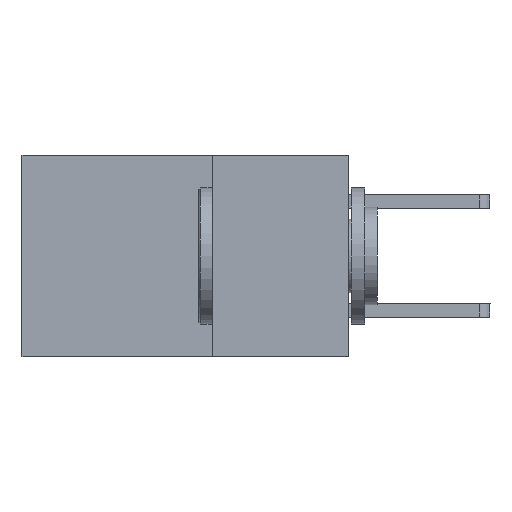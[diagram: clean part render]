
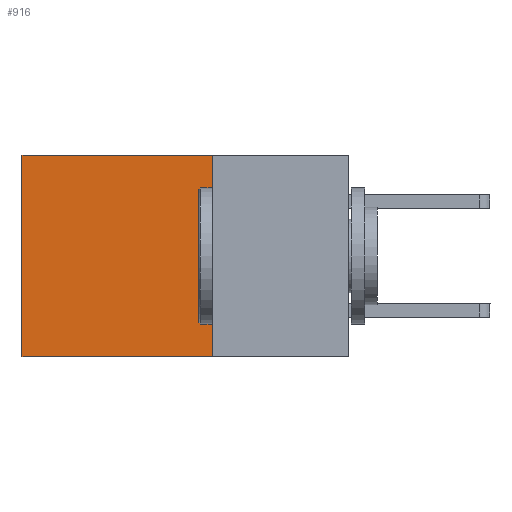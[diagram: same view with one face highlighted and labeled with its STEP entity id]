
A CAD part, left-side view. The second image highlights one B-rep face of the part: STEP entity #916.
In plain terms, the highlighted planar face has unit normal (-1, 0, 0).
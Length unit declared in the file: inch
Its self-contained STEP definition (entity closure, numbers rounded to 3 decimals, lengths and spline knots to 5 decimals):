
#93 = ORIENTED_EDGE ( 'NONE', *, *, #2616, .F. ) ;
#195 = CARTESIAN_POINT ( 'NONE',  ( 0.298, 0.25, 0. ) ) ;
#203 = LINE ( 'NONE', #5521, #3733 ) ;
#425 = VERTEX_POINT ( 'NONE', #1299 ) ;
#738 = DIRECTION ( 'NONE',  ( 0., 0., -1. ) ) ;
#740 = VERTEX_POINT ( 'NONE', #9768 ) ;
#897 = VECTOR ( 'NONE', #2485, 39.37008 ) ;
#916 = ADVANCED_FACE ( 'NONE', ( #6773 ), #8336, .F. ) ;
#918 = VECTOR ( 'NONE', #9414, 39.37008 ) ;
#1045 = DIRECTION ( 'NONE',  ( 0., 0., -1. ) ) ;
#1299 = CARTESIAN_POINT ( 'NONE',  ( 0.298, 0.25, -0.37 ) ) ;
#1540 = CARTESIAN_POINT ( 'NONE',  ( 0.298, 0.25, 0. ) ) ;
#1793 = VECTOR ( 'NONE', #9292, 39.37008 ) ;
#2485 = DIRECTION ( 'NONE',  ( 0., 0., -1. ) ) ;
#2616 = EDGE_CURVE ( 'NONE', #8647, #425, #4197, .T. ) ;
#3731 = CARTESIAN_POINT ( 'NONE',  ( 0.298, 0.25, 0. ) ) ;
#3733 = VECTOR ( 'NONE', #738, 39.37008 ) ;
#3848 = ORIENTED_EDGE ( 'NONE', *, *, #5344, .F. ) ;
#3873 = VERTEX_POINT ( 'NONE', #6506 ) ;
#4197 = LINE ( 'NONE', #195, #897 ) ;
#4497 = ORIENTED_EDGE ( 'NONE', *, *, #9090, .T. ) ;
#4728 = LINE ( 'NONE', #3731, #918 ) ;
#5344 = EDGE_CURVE ( 'NONE', #425, #740, #6095, .T. ) ;
#5521 = CARTESIAN_POINT ( 'NONE',  ( 0.298, 0.6, 0. ) ) ;
#5945 = DIRECTION ( 'NONE',  ( 1., 0., 0. ) ) ;
#6095 = LINE ( 'NONE', #9221, #1793 ) ;
#6506 = CARTESIAN_POINT ( 'NONE',  ( 0.298, 0.6, 0. ) ) ;
#6773 = FACE_OUTER_BOUND ( 'NONE', #7563, .T. ) ;
#7563 = EDGE_LOOP ( 'NONE', ( #10474, #3848, #93, #4497 ) ) ;
#8025 = EDGE_CURVE ( 'NONE', #3873, #740, #203, .T. ) ;
#8336 = PLANE ( 'NONE',  #10372 ) ;
#8373 = CARTESIAN_POINT ( 'NONE',  ( 0.298, 0.25, 0. ) ) ;
#8647 = VERTEX_POINT ( 'NONE', #1540 ) ;
#9090 = EDGE_CURVE ( 'NONE', #8647, #3873, #4728, .T. ) ;
#9221 = CARTESIAN_POINT ( 'NONE',  ( 0.298, 0.25, -0.37 ) ) ;
#9292 = DIRECTION ( 'NONE',  ( 0., 1., 0. ) ) ;
#9414 = DIRECTION ( 'NONE',  ( 0., 1., 0. ) ) ;
#9768 = CARTESIAN_POINT ( 'NONE',  ( 0.298, 0.6, -0.37 ) ) ;
#10372 = AXIS2_PLACEMENT_3D ( 'NONE', #8373, #5945, #1045 ) ;
#10474 = ORIENTED_EDGE ( 'NONE', *, *, #8025, .T. ) ;
